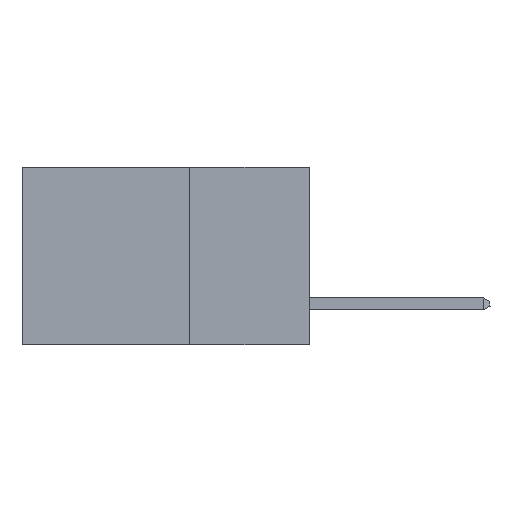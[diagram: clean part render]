
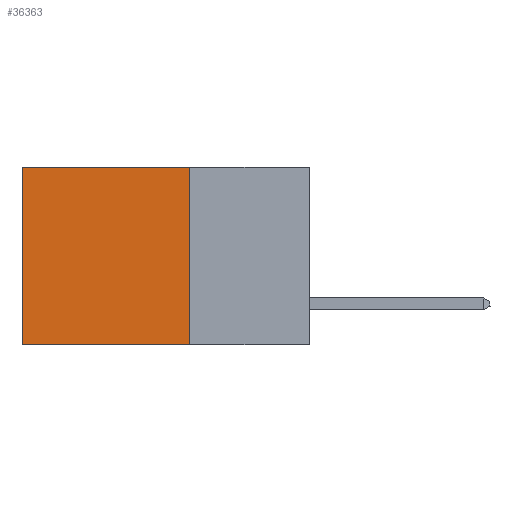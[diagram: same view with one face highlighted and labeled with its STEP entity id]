
A CAD part, left-side view. The second image highlights one B-rep face of the part: STEP entity #36363.
In plain terms, the highlighted planar face has unit normal (-1, 0, 0).
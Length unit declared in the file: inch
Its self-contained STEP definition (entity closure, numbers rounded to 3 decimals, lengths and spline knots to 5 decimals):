
#3127 = VECTOR ( 'NONE', #33558, 39.37008 ) ;
#6359 = CARTESIAN_POINT ( 'NONE',  ( 0.2875, 0.25, 0. ) ) ;
#6557 = DIRECTION ( 'NONE',  ( 0., 1., 0. ) ) ;
#6655 = CARTESIAN_POINT ( 'NONE',  ( 0.2875, 0.6, 0. ) ) ;
#7221 = CARTESIAN_POINT ( 'NONE',  ( 0.2875, 0.25, -0.37 ) ) ;
#11380 = EDGE_CURVE ( 'NONE', #19580, #29978, #22206, .T. ) ;
#12824 = ORIENTED_EDGE ( 'NONE', *, *, #11380, .T. ) ;
#12961 = DIRECTION ( 'NONE',  ( 0., 0., -1. ) ) ;
#13098 = CARTESIAN_POINT ( 'NONE',  ( 0.2875, 0.25, 0. ) ) ;
#14046 = CARTESIAN_POINT ( 'NONE',  ( 0.2875, 0.6, -0.37 ) ) ;
#18324 = VERTEX_POINT ( 'NONE', #24799 ) ;
#19580 = VERTEX_POINT ( 'NONE', #13098 ) ;
#19653 = VERTEX_POINT ( 'NONE', #14046 ) ;
#22117 = AXIS2_PLACEMENT_3D ( 'NONE', #27551, #43032, #12961 ) ;
#22206 = LINE ( 'NONE', #30711, #42310 ) ;
#22257 = EDGE_CURVE ( 'NONE', #29978, #19653, #32113, .T. ) ;
#22295 = VECTOR ( 'NONE', #38330, 39.37008 ) ;
#24799 = CARTESIAN_POINT ( 'NONE',  ( 0.2875, 0.25, -0.37 ) ) ;
#26147 = CARTESIAN_POINT ( 'NONE',  ( 0.2875, 0.6, 0. ) ) ;
#26735 = DIRECTION ( 'NONE',  ( 0., 1., 0. ) ) ;
#27551 = CARTESIAN_POINT ( 'NONE',  ( 0.2875, 0.25, 0. ) ) ;
#27720 = PLANE ( 'NONE',  #22117 ) ;
#28308 = EDGE_CURVE ( 'NONE', #18324, #19653, #40961, .T. ) ;
#29978 = VERTEX_POINT ( 'NONE', #26147 ) ;
#30711 = CARTESIAN_POINT ( 'NONE',  ( 0.2875, 0.25, 0. ) ) ;
#32113 = LINE ( 'NONE', #6655, #3127 ) ;
#32374 = LINE ( 'NONE', #6359, #22295 ) ;
#33558 = DIRECTION ( 'NONE',  ( 0., 0., -1. ) ) ;
#35528 = EDGE_CURVE ( 'NONE', #19580, #18324, #32374, .T. ) ;
#35663 = VECTOR ( 'NONE', #26735, 39.37008 ) ;
#36363 = ADVANCED_FACE ( 'NONE', ( #37586 ), #27720, .F. ) ;
#37586 = FACE_OUTER_BOUND ( 'NONE', #38472, .T. ) ;
#38330 = DIRECTION ( 'NONE',  ( 0., 0., -1. ) ) ;
#38472 = EDGE_LOOP ( 'NONE', ( #45886, #40283, #46679, #12824 ) ) ;
#40283 = ORIENTED_EDGE ( 'NONE', *, *, #28308, .F. ) ;
#40961 = LINE ( 'NONE', #7221, #35663 ) ;
#42310 = VECTOR ( 'NONE', #6557, 39.37008 ) ;
#43032 = DIRECTION ( 'NONE',  ( 1., 0., 0. ) ) ;
#45886 = ORIENTED_EDGE ( 'NONE', *, *, #22257, .T. ) ;
#46679 = ORIENTED_EDGE ( 'NONE', *, *, #35528, .F. ) ;
